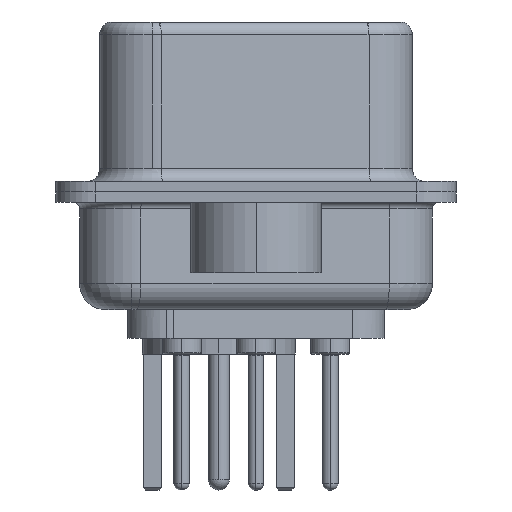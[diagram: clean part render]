
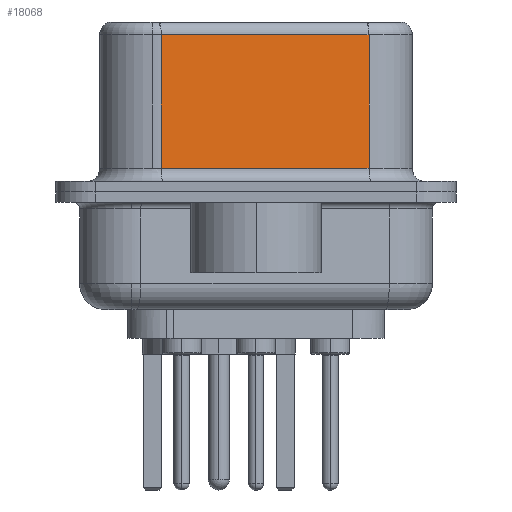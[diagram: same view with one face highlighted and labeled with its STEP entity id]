
A CAD part, left-side view. The second image highlights one B-rep face of the part: STEP entity #18068.
In plain terms, the highlighted planar face has unit normal (-0.985, -0.174, 0).
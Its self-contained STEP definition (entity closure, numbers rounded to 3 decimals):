
#1197 = DIRECTION ( 'NONE',  ( 0.985, 0.174, 0. ) ) ;
#2868 = ORIENTED_EDGE ( 'NONE', *, *, #2971, .F. ) ;
#2971 = EDGE_CURVE ( 'NONE', #4387, #4791, #26691, .T. ) ;
#3034 = EDGE_CURVE ( 'NONE', #12974, #4791, #11797, .T. ) ;
#3534 = EDGE_LOOP ( 'NONE', ( #2868, #7787, #30540, #18228 ) ) ;
#4387 = VERTEX_POINT ( 'NONE', #11563 ) ;
#4776 = DIRECTION ( 'NONE',  ( 0., 0., -1. ) ) ;
#4791 = VERTEX_POINT ( 'NONE', #25168 ) ;
#4811 = EDGE_CURVE ( 'NONE', #4387, #16992, #4956, .T. ) ;
#4956 = LINE ( 'NONE', #18198, #21774 ) ;
#5524 = DIRECTION ( 'NONE',  ( 0., 0., -1. ) ) ;
#5697 = EDGE_CURVE ( 'NONE', #16992, #12974, #25851, .T. ) ;
#7787 = ORIENTED_EDGE ( 'NONE', *, *, #4811, .T. ) ;
#9321 = DIRECTION ( 'NONE',  ( 0.174, -0.985, 0. ) ) ;
#11563 = CARTESIAN_POINT ( 'NONE',  ( 5.132, -4.322, 6.02 ) ) ;
#11601 = FACE_OUTER_BOUND ( 'NONE', #3534, .T. ) ;
#11797 = LINE ( 'NONE', #13111, #17375 ) ;
#11896 = CARTESIAN_POINT ( 'NONE',  ( 3.73, 3.628, 6.52 ) ) ;
#12974 = VERTEX_POINT ( 'NONE', #14513 ) ;
#13111 = CARTESIAN_POINT ( 'NONE',  ( 5.132, -4.322, 0.9 ) ) ;
#13149 = VECTOR ( 'NONE', #4776, 1000. ) ;
#14513 = CARTESIAN_POINT ( 'NONE',  ( 3.73, 3.628, 0.9 ) ) ;
#15563 = CARTESIAN_POINT ( 'NONE',  ( 5.132, -4.322, 6.52 ) ) ;
#16992 = VERTEX_POINT ( 'NONE', #22567 ) ;
#17375 = VECTOR ( 'NONE', #9321, 1000. ) ;
#17956 = DIRECTION ( 'NONE',  ( -0.174, 0.985, 0. ) ) ;
#18068 = ADVANCED_FACE ( 'NONE', ( #11601 ), #29773, .F. ) ;
#18198 = CARTESIAN_POINT ( 'NONE',  ( 5.132, -4.322, 6.02 ) ) ;
#18228 = ORIENTED_EDGE ( 'NONE', *, *, #3034, .T. ) ;
#20583 = DIRECTION ( 'NONE',  ( -0.174, 0.985, 0. ) ) ;
#21774 = VECTOR ( 'NONE', #20583, 1000. ) ;
#22567 = CARTESIAN_POINT ( 'NONE',  ( 3.73, 3.628, 6.02 ) ) ;
#23175 = CARTESIAN_POINT ( 'NONE',  ( 5.132, -4.322, 6.52 ) ) ;
#25168 = CARTESIAN_POINT ( 'NONE',  ( 5.132, -4.322, 0.9 ) ) ;
#25218 = VECTOR ( 'NONE', #5524, 1000. ) ;
#25851 = LINE ( 'NONE', #11896, #13149 ) ;
#26691 = LINE ( 'NONE', #23175, #25218 ) ;
#29183 = AXIS2_PLACEMENT_3D ( 'NONE', #15563, #1197, #17956 ) ;
#29773 = PLANE ( 'NONE',  #29183 ) ;
#30540 = ORIENTED_EDGE ( 'NONE', *, *, #5697, .T. ) ;
